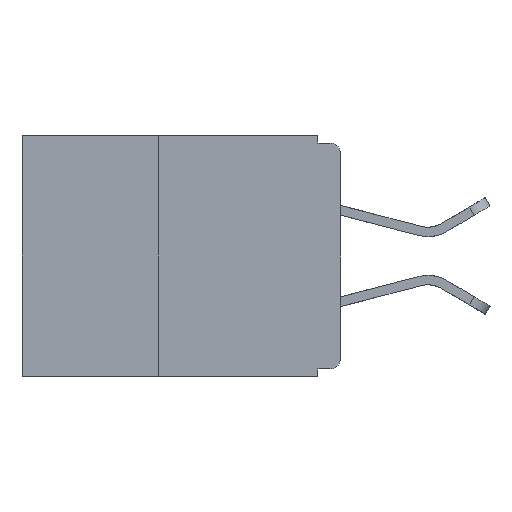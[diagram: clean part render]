
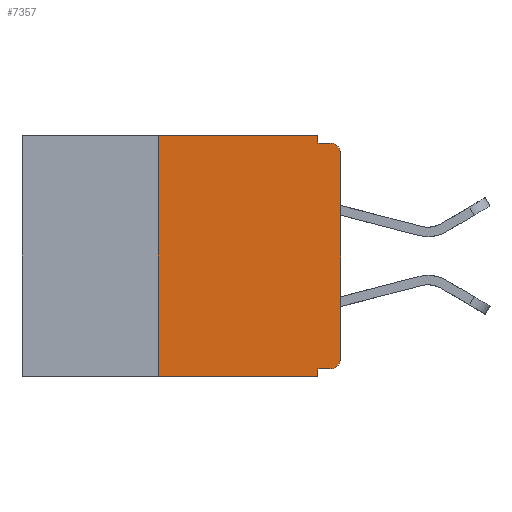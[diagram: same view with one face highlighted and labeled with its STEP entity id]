
A CAD part, left-side view. The second image highlights one B-rep face of the part: STEP entity #7357.
In plain terms, the highlighted planar face has unit normal (-1, 0, 0).
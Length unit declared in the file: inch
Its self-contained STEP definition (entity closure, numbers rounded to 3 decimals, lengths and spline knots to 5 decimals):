
#51 = CARTESIAN_POINT ( 'NONE',  ( 0., 0.25, -0.33 ) ) ;
#81 = DIRECTION ( 'NONE',  ( 0., -1., 0. ) ) ;
#200 = EDGE_CURVE ( 'NONE', #10799, #4927, #576, .T. ) ;
#266 = ORIENTED_EDGE ( 'NONE', *, *, #7485, .T. ) ;
#421 = VECTOR ( 'NONE', #692, 39.37008 ) ;
#461 = EDGE_CURVE ( 'NONE', #10799, #7933, #12461, .T. ) ;
#576 = LINE ( 'NONE', #2560, #4072 ) ;
#689 = DIRECTION ( 'NONE',  ( 0., 0., -1. ) ) ;
#692 = DIRECTION ( 'NONE',  ( 0., -1., 0. ) ) ;
#693 = EDGE_CURVE ( 'NONE', #11600, #11849, #5739, .T. ) ;
#1064 = DIRECTION ( 'NONE',  ( 0., 0., -1. ) ) ;
#1118 = CARTESIAN_POINT ( 'NONE',  ( 0., 0.437, 0. ) ) ;
#1312 = VECTOR ( 'NONE', #5506, 39.37008 ) ;
#1454 = CARTESIAN_POINT ( 'NONE',  ( 0., 0.25, 0. ) ) ;
#1636 = CARTESIAN_POINT ( 'NONE',  ( 0., 0.031, -0.33 ) ) ;
#1714 = CARTESIAN_POINT ( 'NONE',  ( 0., 0., -0.025 ) ) ;
#1869 = CARTESIAN_POINT ( 'NONE',  ( 0., 0.437, -0.33 ) ) ;
#1874 = CARTESIAN_POINT ( 'NONE',  ( 0., 0.25, -0.33 ) ) ;
#1996 = ORIENTED_EDGE ( 'NONE', *, *, #2490, .T. ) ;
#2086 = CIRCLE ( 'NONE', #2980, 0.015 ) ;
#2232 = DIRECTION ( 'NONE',  ( 0., 0., 1. ) ) ;
#2490 = EDGE_CURVE ( 'NONE', #7933, #7138, #8897, .T. ) ;
#2560 = CARTESIAN_POINT ( 'NONE',  ( 0., 0., -0.32 ) ) ;
#2605 = LINE ( 'NONE', #4653, #10250 ) ;
#2749 = VECTOR ( 'NONE', #2232, 39.37008 ) ;
#2980 = AXIS2_PLACEMENT_3D ( 'NONE', #6108, #9981, #8889 ) ;
#3064 = CARTESIAN_POINT ( 'NONE',  ( 0., 0.031, -0.33 ) ) ;
#3152 = DIRECTION ( 'NONE',  ( -1., 0., 0. ) ) ;
#3491 = ORIENTED_EDGE ( 'NONE', *, *, #12644, .F. ) ;
#3850 = DIRECTION ( 'NONE',  ( 1., 0., 0. ) ) ;
#4072 = VECTOR ( 'NONE', #7471, 39.37008 ) ;
#4078 = ORIENTED_EDGE ( 'NONE', *, *, #8968, .F. ) ;
#4261 = VECTOR ( 'NONE', #689, 39.37008 ) ;
#4296 = CARTESIAN_POINT ( 'NONE',  ( 0., 0.015, -0.32 ) ) ;
#4469 = EDGE_CURVE ( 'NONE', #7413, #10075, #2605, .T. ) ;
#4516 = CARTESIAN_POINT ( 'NONE',  ( 0., 0., -0.01 ) ) ;
#4653 = CARTESIAN_POINT ( 'NONE',  ( 0., 0.031, 0. ) ) ;
#4753 = EDGE_CURVE ( 'NONE', #11600, #11428, #11925, .T. ) ;
#4762 = ORIENTED_EDGE ( 'NONE', *, *, #693, .T. ) ;
#4927 = VERTEX_POINT ( 'NONE', #7056 ) ;
#5506 = DIRECTION ( 'NONE',  ( 0., 0., 1. ) ) ;
#5739 = LINE ( 'NONE', #1869, #10016 ) ;
#5953 = CARTESIAN_POINT ( 'NONE',  ( 0., 0.031, -0.01 ) ) ;
#6108 = CARTESIAN_POINT ( 'NONE',  ( 0., 0.015, -0.025 ) ) ;
#6549 = CARTESIAN_POINT ( 'NONE',  ( 0., 0., 0. ) ) ;
#7056 = CARTESIAN_POINT ( 'NONE',  ( 0., 0.031, -0.32 ) ) ;
#7138 = VERTEX_POINT ( 'NONE', #1714 ) ;
#7301 = CARTESIAN_POINT ( 'NONE',  ( 0., 0.015, -0.01 ) ) ;
#7357 = ADVANCED_FACE ( 'NONE', ( #11843 ), #8714, .F. ) ;
#7413 = VERTEX_POINT ( 'NONE', #9829 ) ;
#7471 = DIRECTION ( 'NONE',  ( 0., 1., 0. ) ) ;
#7485 = EDGE_CURVE ( 'NONE', #7138, #12019, #2086, .T. ) ;
#7578 = AXIS2_PLACEMENT_3D ( 'NONE', #8797, #3850, #1064 ) ;
#7758 = ORIENTED_EDGE ( 'NONE', *, *, #4469, .F. ) ;
#7884 = ORIENTED_EDGE ( 'NONE', *, *, #461, .T. ) ;
#7933 = VERTEX_POINT ( 'NONE', #11549 ) ;
#8196 = CARTESIAN_POINT ( 'NONE',  ( 0., 0.015, -0.305 ) ) ;
#8268 = VECTOR ( 'NONE', #81, 39.37008 ) ;
#8649 = DIRECTION ( 'NONE',  ( 0., -1., 0. ) ) ;
#8714 = PLANE ( 'NONE',  #7578 ) ;
#8797 = CARTESIAN_POINT ( 'NONE',  ( 0., 0.437, 0. ) ) ;
#8875 = LINE ( 'NONE', #1118, #8268 ) ;
#8889 = DIRECTION ( 'NONE',  ( 0., 0., -1. ) ) ;
#8897 = LINE ( 'NONE', #6549, #1312 ) ;
#8968 = EDGE_CURVE ( 'NONE', #11428, #7413, #8875, .T. ) ;
#9053 = AXIS2_PLACEMENT_3D ( 'NONE', #8196, #3152, #9062 ) ;
#9062 = DIRECTION ( 'NONE',  ( 0., 0., -1. ) ) ;
#9816 = EDGE_LOOP ( 'NONE', ( #1996, #266, #3491, #7758, #4078, #11489, #4762, #11994, #12621, #7884 ) ) ;
#9829 = CARTESIAN_POINT ( 'NONE',  ( 0., 0.031, 0. ) ) ;
#9872 = LINE ( 'NONE', #4516, #421 ) ;
#9981 = DIRECTION ( 'NONE',  ( -1., 0., 0. ) ) ;
#10016 = VECTOR ( 'NONE', #8649, 39.37008 ) ;
#10075 = VERTEX_POINT ( 'NONE', #5953 ) ;
#10250 = VECTOR ( 'NONE', #11409, 39.37008 ) ;
#10799 = VERTEX_POINT ( 'NONE', #4296 ) ;
#10872 = EDGE_CURVE ( 'NONE', #4927, #11849, #11911, .T. ) ;
#11409 = DIRECTION ( 'NONE',  ( 0., 0., -1. ) ) ;
#11428 = VERTEX_POINT ( 'NONE', #1454 ) ;
#11489 = ORIENTED_EDGE ( 'NONE', *, *, #4753, .F. ) ;
#11549 = CARTESIAN_POINT ( 'NONE',  ( 0., 0., -0.305 ) ) ;
#11600 = VERTEX_POINT ( 'NONE', #1874 ) ;
#11843 = FACE_OUTER_BOUND ( 'NONE', #9816, .T. ) ;
#11849 = VERTEX_POINT ( 'NONE', #3064 ) ;
#11911 = LINE ( 'NONE', #1636, #4261 ) ;
#11925 = LINE ( 'NONE', #51, #2749 ) ;
#11994 = ORIENTED_EDGE ( 'NONE', *, *, #10872, .F. ) ;
#12019 = VERTEX_POINT ( 'NONE', #7301 ) ;
#12461 = CIRCLE ( 'NONE', #9053, 0.015 ) ;
#12621 = ORIENTED_EDGE ( 'NONE', *, *, #200, .F. ) ;
#12644 = EDGE_CURVE ( 'NONE', #10075, #12019, #9872, .T. ) ;
